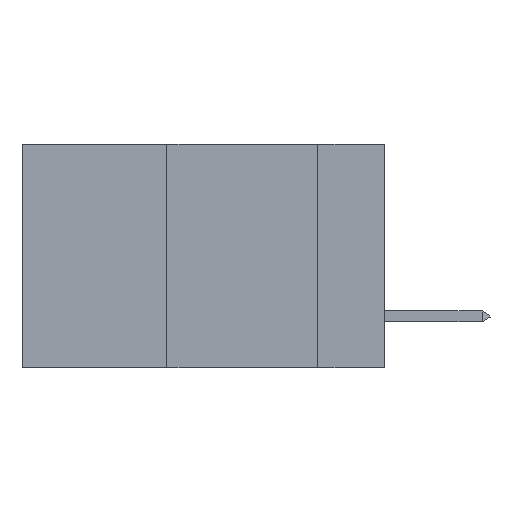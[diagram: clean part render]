
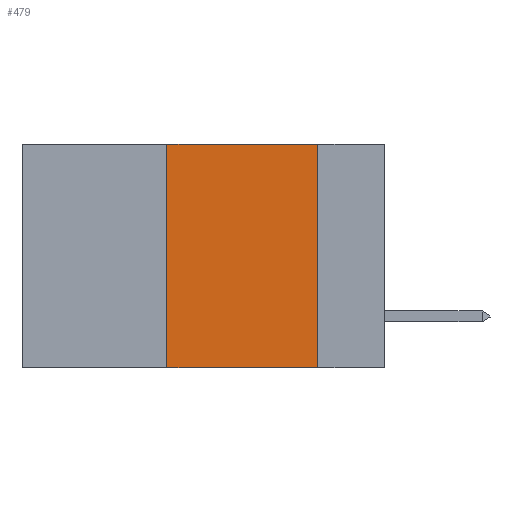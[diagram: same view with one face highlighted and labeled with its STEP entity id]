
A CAD part, left-side view. The second image highlights one B-rep face of the part: STEP entity #479.
In plain terms, the highlighted planar face has unit normal (-1, 0, 0).
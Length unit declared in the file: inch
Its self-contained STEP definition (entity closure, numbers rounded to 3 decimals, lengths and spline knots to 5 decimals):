
#144 = DIRECTION ( 'NONE',  ( 0., 0., 1. ) ) ;
#237 = VERTEX_POINT ( 'NONE', #11489 ) ;
#479 = ADVANCED_FACE ( 'NONE', ( #4469 ), #12367, .F. ) ;
#1532 = DIRECTION ( 'NONE',  ( 0., -1., 0. ) ) ;
#1716 = EDGE_CURVE ( 'NONE', #3283, #237, #11222, .T. ) ;
#1777 = CARTESIAN_POINT ( 'NONE',  ( 0., 0.11, 0. ) ) ;
#1839 = ORIENTED_EDGE ( 'NONE', *, *, #10771, .F. ) ;
#3097 = DIRECTION ( 'NONE',  ( 0., 0., -1. ) ) ;
#3283 = VERTEX_POINT ( 'NONE', #3757 ) ;
#3757 = CARTESIAN_POINT ( 'NONE',  ( 0., 0.36, -0.37 ) ) ;
#4469 = FACE_OUTER_BOUND ( 'NONE', #11473, .T. ) ;
#5306 = CARTESIAN_POINT ( 'NONE',  ( 0., 0.11, 0. ) ) ;
#5767 = VECTOR ( 'NONE', #3097, 39.37008 ) ;
#5861 = CARTESIAN_POINT ( 'NONE',  ( 0., 0.6, 0. ) ) ;
#5998 = LINE ( 'NONE', #8268, #11603 ) ;
#6213 = ORIENTED_EDGE ( 'NONE', *, *, #8421, .F. ) ;
#7087 = DIRECTION ( 'NONE',  ( 0., -1., 0. ) ) ;
#7848 = DIRECTION ( 'NONE',  ( 0., 0., -1. ) ) ;
#7891 = ORIENTED_EDGE ( 'NONE', *, *, #1716, .T. ) ;
#8268 = CARTESIAN_POINT ( 'NONE',  ( 0., 0.6, 0. ) ) ;
#8380 = LINE ( 'NONE', #5306, #5767 ) ;
#8421 = EDGE_CURVE ( 'NONE', #9282, #237, #8380, .T. ) ;
#8481 = CARTESIAN_POINT ( 'NONE',  ( 0., 0.6, -0.37 ) ) ;
#8496 = ORIENTED_EDGE ( 'NONE', *, *, #12287, .F. ) ;
#9048 = CARTESIAN_POINT ( 'NONE',  ( 0., 0.36, 0. ) ) ;
#9120 = DIRECTION ( 'NONE',  ( 1., 0., 0. ) ) ;
#9282 = VERTEX_POINT ( 'NONE', #1777 ) ;
#10482 = VERTEX_POINT ( 'NONE', #11724 ) ;
#10771 = EDGE_CURVE ( 'NONE', #3283, #10482, #11812, .T. ) ;
#11222 = LINE ( 'NONE', #8481, #14339 ) ;
#11473 = EDGE_LOOP ( 'NONE', ( #6213, #8496, #1839, #7891 ) ) ;
#11489 = CARTESIAN_POINT ( 'NONE',  ( 0., 0.11, -0.37 ) ) ;
#11603 = VECTOR ( 'NONE', #7087, 39.37008 ) ;
#11724 = CARTESIAN_POINT ( 'NONE',  ( 0., 0.36, 0. ) ) ;
#11812 = LINE ( 'NONE', #9048, #13010 ) ;
#12287 = EDGE_CURVE ( 'NONE', #10482, #9282, #5998, .T. ) ;
#12367 = PLANE ( 'NONE',  #14344 ) ;
#13010 = VECTOR ( 'NONE', #144, 39.37008 ) ;
#14339 = VECTOR ( 'NONE', #1532, 39.37008 ) ;
#14344 = AXIS2_PLACEMENT_3D ( 'NONE', #5861, #9120, #7848 ) ;
